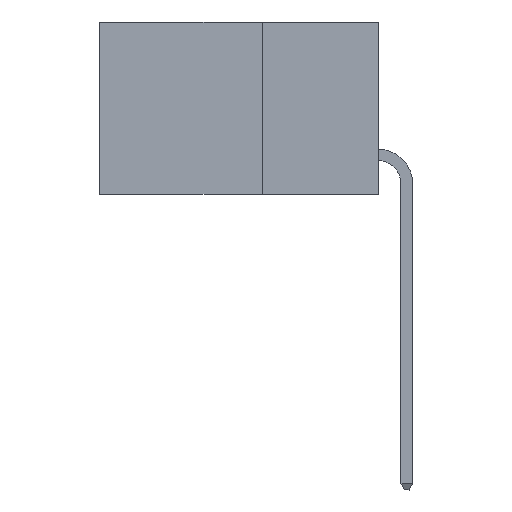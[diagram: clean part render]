
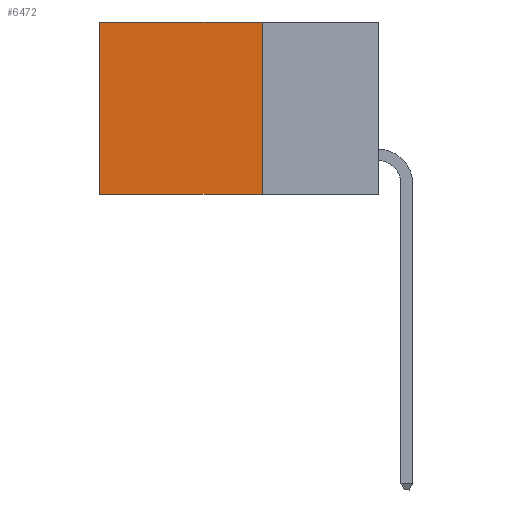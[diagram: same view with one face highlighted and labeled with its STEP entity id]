
A CAD part, left-side view. The second image highlights one B-rep face of the part: STEP entity #6472.
In plain terms, the highlighted planar face has unit normal (-1, 0, 0).
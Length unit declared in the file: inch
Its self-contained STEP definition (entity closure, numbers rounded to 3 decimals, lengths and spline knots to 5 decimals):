
#396 = VERTEX_POINT ( 'NONE', #25961 ) ;
#1830 = CARTESIAN_POINT ( 'NONE',  ( 0.298, 0.25, 0. ) ) ;
#1926 = VERTEX_POINT ( 'NONE', #14057 ) ;
#5016 = FACE_OUTER_BOUND ( 'NONE', #6931, .T. ) ;
#5074 = CARTESIAN_POINT ( 'NONE',  ( 0.298, 0.25, 0. ) ) ;
#6472 = ADVANCED_FACE ( 'NONE', ( #5016 ), #14749, .F. ) ;
#6586 = LINE ( 'NONE', #23061, #9004 ) ;
#6931 = EDGE_LOOP ( 'NONE', ( #18094, #22603, #14665, #17619 ) ) ;
#8489 = DIRECTION ( 'NONE',  ( 0., 0., -1. ) ) ;
#8971 = DIRECTION ( 'NONE',  ( 0., 1., 0. ) ) ;
#9004 = VECTOR ( 'NONE', #16311, 39.37008 ) ;
#9147 = DIRECTION ( 'NONE',  ( 0., 0., -1. ) ) ;
#9382 = EDGE_CURVE ( 'NONE', #396, #24533, #16614, .T. ) ;
#9446 = EDGE_CURVE ( 'NONE', #1926, #24533, #6586, .T. ) ;
#9803 = DIRECTION ( 'NONE',  ( 0., 0., -1. ) ) ;
#9933 = AXIS2_PLACEMENT_3D ( 'NONE', #17693, #13389, #9147 ) ;
#11087 = VECTOR ( 'NONE', #9803, 39.37008 ) ;
#13320 = LINE ( 'NONE', #28837, #25919 ) ;
#13389 = DIRECTION ( 'NONE',  ( 1., 0., 0. ) ) ;
#14057 = CARTESIAN_POINT ( 'NONE',  ( 0.298, 0.25, -0.37 ) ) ;
#14665 = ORIENTED_EDGE ( 'NONE', *, *, #14803, .F. ) ;
#14749 = PLANE ( 'NONE',  #9933 ) ;
#14803 = EDGE_CURVE ( 'NONE', #27830, #1926, #26080, .T. ) ;
#16311 = DIRECTION ( 'NONE',  ( 0., 1., 0. ) ) ;
#16614 = LINE ( 'NONE', #21842, #20850 ) ;
#17619 = ORIENTED_EDGE ( 'NONE', *, *, #28525, .T. ) ;
#17693 = CARTESIAN_POINT ( 'NONE',  ( 0.298, 0.25, 0. ) ) ;
#18094 = ORIENTED_EDGE ( 'NONE', *, *, #9382, .T. ) ;
#20015 = CARTESIAN_POINT ( 'NONE',  ( 0.298, 0.6, -0.37 ) ) ;
#20850 = VECTOR ( 'NONE', #8489, 39.37008 ) ;
#21842 = CARTESIAN_POINT ( 'NONE',  ( 0.298, 0.6, 0. ) ) ;
#22603 = ORIENTED_EDGE ( 'NONE', *, *, #9446, .F. ) ;
#23061 = CARTESIAN_POINT ( 'NONE',  ( 0.298, 0.25, -0.37 ) ) ;
#24533 = VERTEX_POINT ( 'NONE', #20015 ) ;
#25919 = VECTOR ( 'NONE', #8971, 39.37008 ) ;
#25961 = CARTESIAN_POINT ( 'NONE',  ( 0.298, 0.6, 0. ) ) ;
#26080 = LINE ( 'NONE', #5074, #11087 ) ;
#27830 = VERTEX_POINT ( 'NONE', #1830 ) ;
#28525 = EDGE_CURVE ( 'NONE', #27830, #396, #13320, .T. ) ;
#28837 = CARTESIAN_POINT ( 'NONE',  ( 0.298, 0.25, 0. ) ) ;
